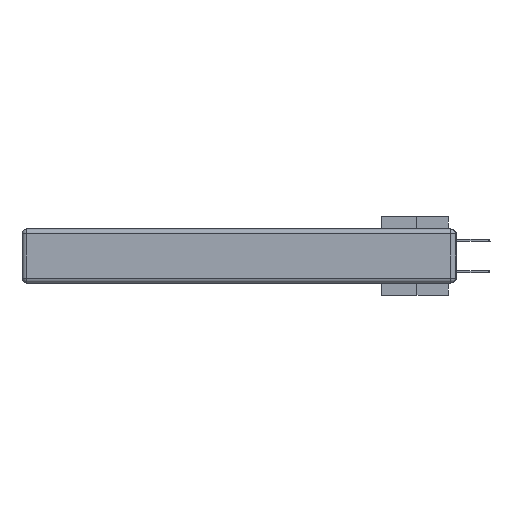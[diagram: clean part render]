
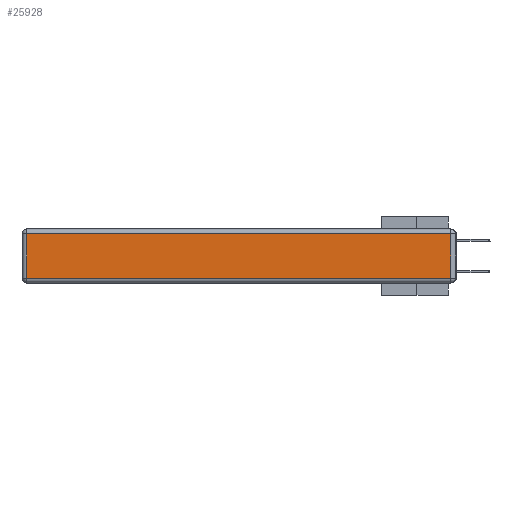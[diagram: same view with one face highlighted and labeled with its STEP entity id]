
A CAD part, left-side view. The second image highlights one B-rep face of the part: STEP entity #25928.
In plain terms, the highlighted planar face has unit normal (-1, 0, 0).
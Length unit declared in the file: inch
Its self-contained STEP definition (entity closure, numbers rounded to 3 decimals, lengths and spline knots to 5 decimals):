
#164 = ORIENTED_EDGE ( 'NONE', *, *, #2684, .T. ) ;
#788 = DIRECTION ( 'NONE',  ( 0., 0., -1. ) ) ;
#2684 = EDGE_CURVE ( 'NONE', #12940, #6190, #20504, .T. ) ;
#3026 = VECTOR ( 'NONE', #788, 39.37008 ) ;
#6190 = VERTEX_POINT ( 'NONE', #23843 ) ;
#6303 = VECTOR ( 'NONE', #20964, 39.37008 ) ;
#6753 = DIRECTION ( 'NONE',  ( 0., 1., 0. ) ) ;
#6810 = EDGE_CURVE ( 'NONE', #9533, #12940, #28659, .T. ) ;
#7434 = VERTEX_POINT ( 'NONE', #29859 ) ;
#9533 = VERTEX_POINT ( 'NONE', #15273 ) ;
#9905 = EDGE_CURVE ( 'NONE', #7434, #9533, #29882, .T. ) ;
#10076 = DIRECTION ( 'NONE',  ( 0., -1., 0. ) ) ;
#10992 = CARTESIAN_POINT ( 'NONE',  ( 0., 2.72, -0.343 ) ) ;
#11349 = ORIENTED_EDGE ( 'NONE', *, *, #17516, .T. ) ;
#12940 = VERTEX_POINT ( 'NONE', #30345 ) ;
#15273 = CARTESIAN_POINT ( 'NONE',  ( 0., 2.72, -0.313 ) ) ;
#15816 = CARTESIAN_POINT ( 'NONE',  ( 0., 0.03, -0.343 ) ) ;
#16535 = ORIENTED_EDGE ( 'NONE', *, *, #9905, .T. ) ;
#17516 = EDGE_CURVE ( 'NONE', #6190, #7434, #25620, .T. ) ;
#17872 = CARTESIAN_POINT ( 'NONE',  ( 0., 0., -0.343 ) ) ;
#19782 = CARTESIAN_POINT ( 'NONE',  ( 0., 0., -0.313 ) ) ;
#20065 = DIRECTION ( 'NONE',  ( 0., 0., 1. ) ) ;
#20345 = ORIENTED_EDGE ( 'NONE', *, *, #6810, .T. ) ;
#20504 = LINE ( 'NONE', #15816, #6303 ) ;
#20964 = DIRECTION ( 'NONE',  ( 0., 0., 1. ) ) ;
#22385 = FACE_OUTER_BOUND ( 'NONE', #29717, .T. ) ;
#23843 = CARTESIAN_POINT ( 'NONE',  ( 0., 0.03, -0.03 ) ) ;
#24851 = PLANE ( 'NONE',  #26574 ) ;
#25620 = LINE ( 'NONE', #28141, #29767 ) ;
#25928 = ADVANCED_FACE ( 'NONE', ( #22385 ), #24851, .T. ) ;
#26574 = AXIS2_PLACEMENT_3D ( 'NONE', #17872, #27344, #20065 ) ;
#27344 = DIRECTION ( 'NONE',  ( -1., 0., 0. ) ) ;
#28141 = CARTESIAN_POINT ( 'NONE',  ( 0., 2.75, -0.03 ) ) ;
#28659 = LINE ( 'NONE', #19782, #29900 ) ;
#29717 = EDGE_LOOP ( 'NONE', ( #20345, #164, #11349, #16535 ) ) ;
#29767 = VECTOR ( 'NONE', #6753, 39.37008 ) ;
#29859 = CARTESIAN_POINT ( 'NONE',  ( 0., 2.72, -0.03 ) ) ;
#29882 = LINE ( 'NONE', #10992, #3026 ) ;
#29900 = VECTOR ( 'NONE', #10076, 39.37008 ) ;
#30345 = CARTESIAN_POINT ( 'NONE',  ( 0., 0.03, -0.313 ) ) ;
